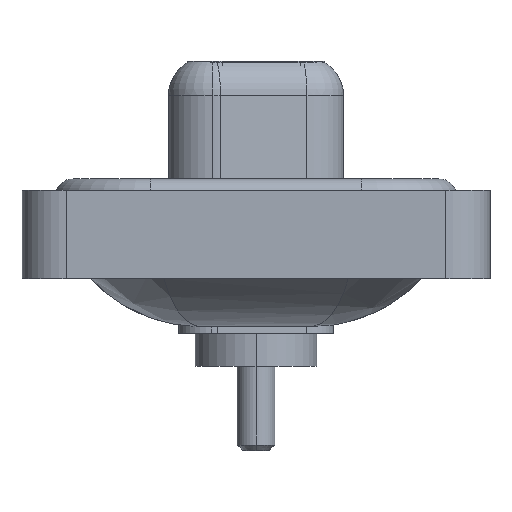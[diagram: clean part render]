
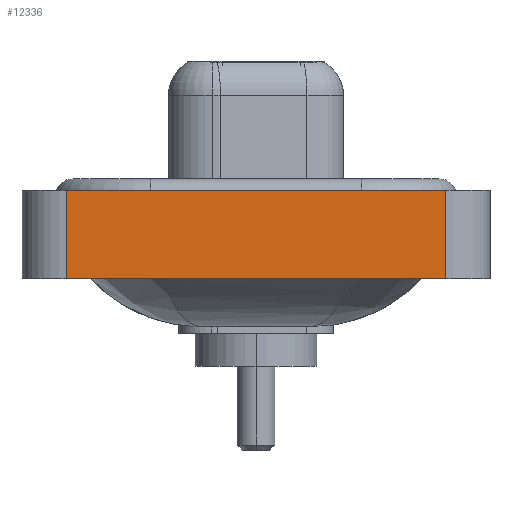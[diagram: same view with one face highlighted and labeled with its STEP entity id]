
A CAD part, left-side view. The second image highlights one B-rep face of the part: STEP entity #12336.
In plain terms, the highlighted planar face has unit normal (-1, 0, 0).
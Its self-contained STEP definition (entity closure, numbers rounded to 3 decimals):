
#489 = VERTEX_POINT ( 'NONE', #11378 ) ;
#1444 = DIRECTION ( 'NONE',  ( 0., 0., 1. ) ) ;
#1646 = CARTESIAN_POINT ( 'NONE',  ( -7.25, 8.55, -3.6 ) ) ;
#2073 = LINE ( 'NONE', #10967, #14578 ) ;
#2636 = VERTEX_POINT ( 'NONE', #1646 ) ;
#3680 = CARTESIAN_POINT ( 'NONE',  ( -7.25, -8.55, -3.6 ) ) ;
#4597 = CARTESIAN_POINT ( 'NONE',  ( -7.25, -8.55, -3.6 ) ) ;
#4764 = AXIS2_PLACEMENT_3D ( 'NONE', #15730, #11860, #1444 ) ;
#6891 = VECTOR ( 'NONE', #7853, 1000. ) ;
#6987 = PLANE ( 'NONE',  #4764 ) ;
#7078 = LINE ( 'NONE', #4597, #15667 ) ;
#7853 = DIRECTION ( 'NONE',  ( 0., 0., 1. ) ) ;
#9518 = DIRECTION ( 'NONE',  ( 0., -1., 0. ) ) ;
#10423 = CARTESIAN_POINT ( 'NONE',  ( -7.25, -8.55, -3.6 ) ) ;
#10643 = EDGE_CURVE ( 'NONE', #14520, #489, #7078, .T. ) ;
#10682 = ORIENTED_EDGE ( 'NONE', *, *, #16005, .F. ) ;
#10694 = CARTESIAN_POINT ( 'NONE',  ( -7.25, 8.55, -3.6 ) ) ;
#10939 = DIRECTION ( 'NONE',  ( 0., 0., 1. ) ) ;
#10967 = CARTESIAN_POINT ( 'NONE',  ( -7.25, -8.55, 0.4 ) ) ;
#11378 = CARTESIAN_POINT ( 'NONE',  ( -7.25, -8.55, 0.4 ) ) ;
#11770 = EDGE_CURVE ( 'NONE', #2636, #14520, #15403, .T. ) ;
#11798 = DIRECTION ( 'NONE',  ( 0., -1., 0. ) ) ;
#11803 = LINE ( 'NONE', #10694, #6891 ) ;
#11860 = DIRECTION ( 'NONE',  ( -1., 0., 0. ) ) ;
#12336 = ADVANCED_FACE ( 'NONE', ( #14528 ), #6987, .T. ) ;
#14081 = ORIENTED_EDGE ( 'NONE', *, *, #10643, .T. ) ;
#14189 = EDGE_LOOP ( 'NONE', ( #14081, #15896, #10682, #16074 ) ) ;
#14520 = VERTEX_POINT ( 'NONE', #10423 ) ;
#14528 = FACE_OUTER_BOUND ( 'NONE', #14189, .T. ) ;
#14578 = VECTOR ( 'NONE', #9518, 1000. ) ;
#14829 = CARTESIAN_POINT ( 'NONE',  ( -7.25, 8.55, 0.4 ) ) ;
#15131 = VECTOR ( 'NONE', #11798, 1000. ) ;
#15403 = LINE ( 'NONE', #3680, #15131 ) ;
#15667 = VECTOR ( 'NONE', #10939, 1000. ) ;
#15730 = CARTESIAN_POINT ( 'NONE',  ( -7.25, -8.55, -3.6 ) ) ;
#15759 = EDGE_CURVE ( 'NONE', #16740, #489, #2073, .T. ) ;
#15896 = ORIENTED_EDGE ( 'NONE', *, *, #15759, .F. ) ;
#16005 = EDGE_CURVE ( 'NONE', #2636, #16740, #11803, .T. ) ;
#16074 = ORIENTED_EDGE ( 'NONE', *, *, #11770, .T. ) ;
#16740 = VERTEX_POINT ( 'NONE', #14829 ) ;
